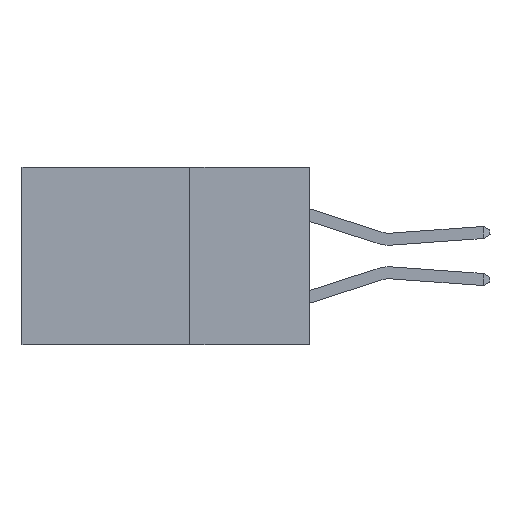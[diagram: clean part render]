
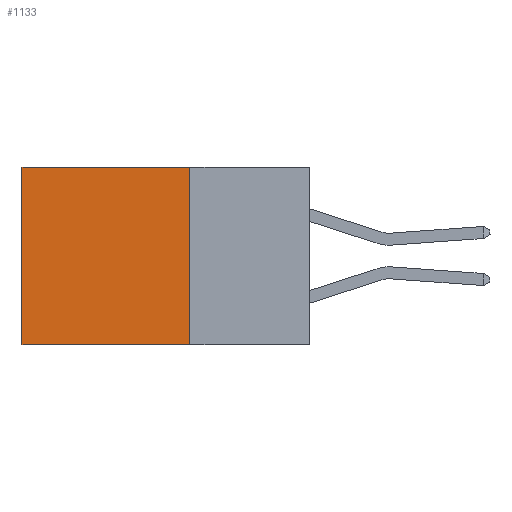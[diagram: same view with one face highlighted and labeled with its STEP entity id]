
A CAD part, left-side view. The second image highlights one B-rep face of the part: STEP entity #1133.
In plain terms, the highlighted planar face has unit normal (-1, 0, 0).
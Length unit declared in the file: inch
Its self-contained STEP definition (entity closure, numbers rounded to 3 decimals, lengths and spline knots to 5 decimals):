
#117 = LINE ( 'NONE', #4741, #10934 ) ;
#237 = CARTESIAN_POINT ( 'NONE',  ( 0.2615, 0.25, -0.37 ) ) ;
#366 = LINE ( 'NONE', #4976, #11879 ) ;
#1133 = ADVANCED_FACE ( 'NONE', ( #6142 ), #10752, .F. ) ;
#1326 = CARTESIAN_POINT ( 'NONE',  ( 0.2615, 0.25, -0.37 ) ) ;
#1587 = ORIENTED_EDGE ( 'NONE', *, *, #6937, .F. ) ;
#2358 = VERTEX_POINT ( 'NONE', #7721 ) ;
#2969 = CARTESIAN_POINT ( 'NONE',  ( 0.2615, 0.25, -0.37 ) ) ;
#3183 = VERTEX_POINT ( 'NONE', #7685 ) ;
#3419 = ORIENTED_EDGE ( 'NONE', *, *, #12683, .F. ) ;
#4741 = CARTESIAN_POINT ( 'NONE',  ( 0.2615, 0.25, -0.37 ) ) ;
#4976 = CARTESIAN_POINT ( 'NONE',  ( 0.2615, 0.25, 0. ) ) ;
#5378 = DIRECTION ( 'NONE',  ( 0., 0., -1. ) ) ;
#5594 = EDGE_CURVE ( 'NONE', #3183, #2358, #13543, .T. ) ;
#6142 = FACE_OUTER_BOUND ( 'NONE', #12078, .T. ) ;
#6486 = EDGE_CURVE ( 'NONE', #6832, #3183, #366, .T. ) ;
#6832 = VERTEX_POINT ( 'NONE', #12769 ) ;
#6937 = EDGE_CURVE ( 'NONE', #7769, #2358, #117, .T. ) ;
#6979 = DIRECTION ( 'NONE',  ( 0., 0., -1. ) ) ;
#7685 = CARTESIAN_POINT ( 'NONE',  ( 0.2615, 0.6, 0. ) ) ;
#7721 = CARTESIAN_POINT ( 'NONE',  ( 0.2615, 0.6, -0.37 ) ) ;
#7769 = VERTEX_POINT ( 'NONE', #1326 ) ;
#8501 = DIRECTION ( 'NONE',  ( 0., 0., -1. ) ) ;
#8575 = CARTESIAN_POINT ( 'NONE',  ( 0.2615, 0.6, -0.37 ) ) ;
#9369 = DIRECTION ( 'NONE',  ( 0., 1., 0. ) ) ;
#10686 = ORIENTED_EDGE ( 'NONE', *, *, #6486, .T. ) ;
#10752 = PLANE ( 'NONE',  #10838 ) ;
#10838 = AXIS2_PLACEMENT_3D ( 'NONE', #237, #12959, #6979 ) ;
#10934 = VECTOR ( 'NONE', #9369, 39.37008 ) ;
#11061 = LINE ( 'NONE', #2969, #12987 ) ;
#11879 = VECTOR ( 'NONE', #14222, 39.37008 ) ;
#12078 = EDGE_LOOP ( 'NONE', ( #13038, #1587, #3419, #10686 ) ) ;
#12683 = EDGE_CURVE ( 'NONE', #6832, #7769, #11061, .T. ) ;
#12769 = CARTESIAN_POINT ( 'NONE',  ( 0.2615, 0.25, 0. ) ) ;
#12959 = DIRECTION ( 'NONE',  ( 1., 0., 0. ) ) ;
#12987 = VECTOR ( 'NONE', #5378, 39.37008 ) ;
#13038 = ORIENTED_EDGE ( 'NONE', *, *, #5594, .T. ) ;
#13543 = LINE ( 'NONE', #8575, #14089 ) ;
#14089 = VECTOR ( 'NONE', #8501, 39.37008 ) ;
#14222 = DIRECTION ( 'NONE',  ( 0., 1., 0. ) ) ;
